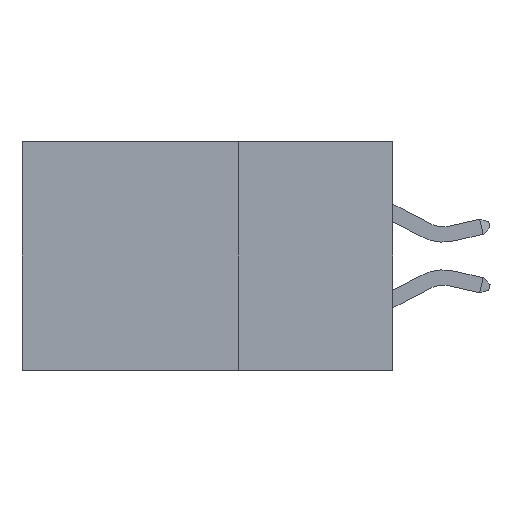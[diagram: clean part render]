
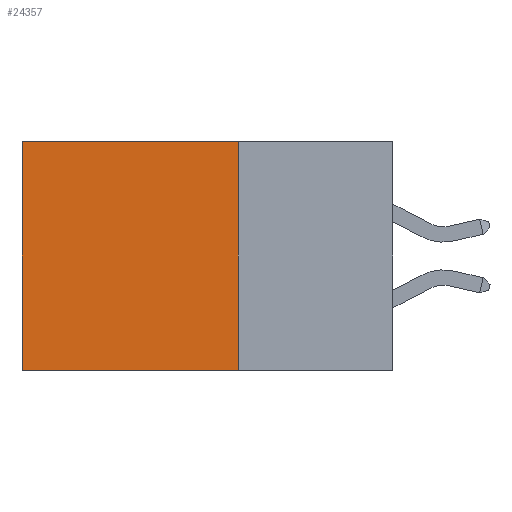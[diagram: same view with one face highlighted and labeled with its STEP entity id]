
A CAD part, left-side view. The second image highlights one B-rep face of the part: STEP entity #24357.
In plain terms, the highlighted planar face has unit normal (-1, 0, 0).
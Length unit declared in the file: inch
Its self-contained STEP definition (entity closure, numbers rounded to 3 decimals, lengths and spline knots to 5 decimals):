
#185 = VECTOR ( 'NONE', #9069, 39.37008 ) ;
#2629 = PLANE ( 'NONE',  #19959 ) ;
#3012 = VERTEX_POINT ( 'NONE', #11878 ) ;
#3132 = VECTOR ( 'NONE', #29447, 39.37008 ) ;
#3267 = EDGE_CURVE ( 'NONE', #10286, #10613, #19020, .T. ) ;
#4534 = EDGE_CURVE ( 'NONE', #10613, #7174, #27277, .T. ) ;
#5023 = DIRECTION ( 'NONE',  ( 1., 0., 0. ) ) ;
#5481 = CARTESIAN_POINT ( 'NONE',  ( 0.2875, 0.6, 0. ) ) ;
#5944 = EDGE_CURVE ( 'NONE', #10286, #3012, #24683, .T. ) ;
#7174 = VERTEX_POINT ( 'NONE', #10171 ) ;
#7239 = FACE_OUTER_BOUND ( 'NONE', #14107, .T. ) ;
#9069 = DIRECTION ( 'NONE',  ( 0., 0., -1. ) ) ;
#10171 = CARTESIAN_POINT ( 'NONE',  ( 0.2875, 0.6, -0.37 ) ) ;
#10286 = VERTEX_POINT ( 'NONE', #20378 ) ;
#10385 = ORIENTED_EDGE ( 'NONE', *, *, #3267, .T. ) ;
#10613 = VERTEX_POINT ( 'NONE', #5481 ) ;
#11878 = CARTESIAN_POINT ( 'NONE',  ( 0.2875, 0.25, -0.37 ) ) ;
#12787 = CARTESIAN_POINT ( 'NONE',  ( 0.2875, 0.25, 0. ) ) ;
#12924 = VECTOR ( 'NONE', #19730, 39.37008 ) ;
#13689 = CARTESIAN_POINT ( 'NONE',  ( 0.2875, 0.25, 0. ) ) ;
#14107 = EDGE_LOOP ( 'NONE', ( #23197, #22660, #22312, #10385 ) ) ;
#19020 = LINE ( 'NONE', #12787, #12924 ) ;
#19730 = DIRECTION ( 'NONE',  ( 0., 1., 0. ) ) ;
#19959 = AXIS2_PLACEMENT_3D ( 'NONE', #27986, #5023, #21124 ) ;
#20274 = CARTESIAN_POINT ( 'NONE',  ( 0.2875, 0.6, 0. ) ) ;
#20378 = CARTESIAN_POINT ( 'NONE',  ( 0.2875, 0.25, 0. ) ) ;
#21122 = VECTOR ( 'NONE', #24906, 39.37008 ) ;
#21124 = DIRECTION ( 'NONE',  ( 0., 0., -1. ) ) ;
#21659 = EDGE_CURVE ( 'NONE', #3012, #7174, #26174, .T. ) ;
#22312 = ORIENTED_EDGE ( 'NONE', *, *, #5944, .F. ) ;
#22571 = CARTESIAN_POINT ( 'NONE',  ( 0.2875, 0.25, -0.37 ) ) ;
#22660 = ORIENTED_EDGE ( 'NONE', *, *, #21659, .F. ) ;
#23197 = ORIENTED_EDGE ( 'NONE', *, *, #4534, .T. ) ;
#24357 = ADVANCED_FACE ( 'NONE', ( #7239 ), #2629, .F. ) ;
#24683 = LINE ( 'NONE', #13689, #185 ) ;
#24906 = DIRECTION ( 'NONE',  ( 0., 0., -1. ) ) ;
#26174 = LINE ( 'NONE', #22571, #3132 ) ;
#27277 = LINE ( 'NONE', #20274, #21122 ) ;
#27986 = CARTESIAN_POINT ( 'NONE',  ( 0.2875, 0.25, 0. ) ) ;
#29447 = DIRECTION ( 'NONE',  ( 0., 1., 0. ) ) ;
